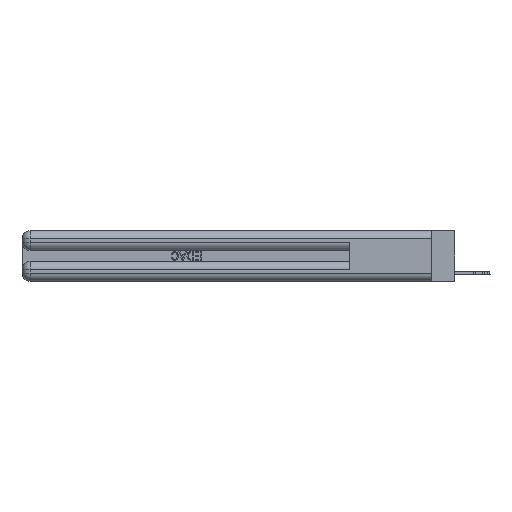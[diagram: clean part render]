
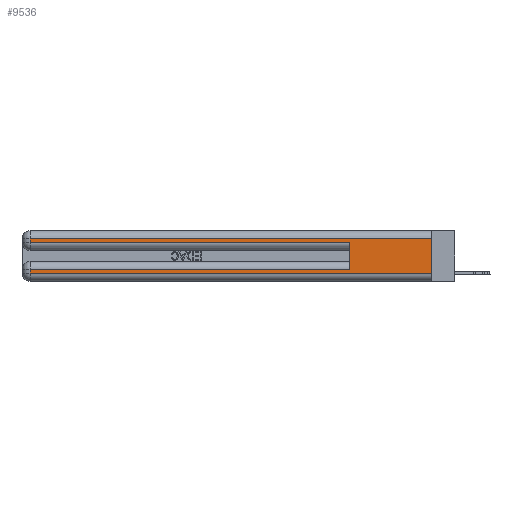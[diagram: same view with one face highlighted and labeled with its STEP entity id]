
A CAD part, left-side view. The second image highlights one B-rep face of the part: STEP entity #9536.
In plain terms, the highlighted planar face has unit normal (-1, 0, 0).
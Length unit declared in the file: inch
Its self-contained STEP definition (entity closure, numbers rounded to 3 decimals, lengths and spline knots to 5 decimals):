
#325 = DIRECTION ( 'NONE',  ( 0., -1., 0. ) ) ;
#1026 = VERTEX_POINT ( 'NONE', #5305 ) ;
#1124 = VERTEX_POINT ( 'NONE', #21292 ) ;
#1587 = CARTESIAN_POINT ( 'NONE',  ( 0., 2.94, 0.37 ) ) ;
#1974 = AXIS2_PLACEMENT_3D ( 'NONE', #2310, #13023, #29664 ) ;
#2194 = EDGE_CURVE ( 'NONE', #16568, #1026, #15857, .T. ) ;
#2310 = CARTESIAN_POINT ( 'NONE',  ( 0., 0., 0.37 ) ) ;
#2945 = LINE ( 'NONE', #22419, #12082 ) ;
#3124 = VERTEX_POINT ( 'NONE', #22089 ) ;
#4169 = ORIENTED_EDGE ( 'NONE', *, *, #14176, .T. ) ;
#4468 = VECTOR ( 'NONE', #27201, 39.37008 ) ;
#5286 = CARTESIAN_POINT ( 'NONE',  ( 0., 2.94, 0.085 ) ) ;
#5305 = CARTESIAN_POINT ( 'NONE',  ( 0., 0.6, 0.285 ) ) ;
#5596 = EDGE_CURVE ( 'NONE', #6558, #3124, #19671, .T. ) ;
#5661 = EDGE_CURVE ( 'NONE', #9516, #1124, #25423, .T. ) ;
#6558 = VERTEX_POINT ( 'NONE', #21133 ) ;
#6864 = ORIENTED_EDGE ( 'NONE', *, *, #15532, .T. ) ;
#7749 = PLANE ( 'NONE',  #1974 ) ;
#7805 = ORIENTED_EDGE ( 'NONE', *, *, #5661, .T. ) ;
#8416 = CARTESIAN_POINT ( 'NONE',  ( 0., 0., 0.06 ) ) ;
#9507 = LINE ( 'NONE', #20895, #17770 ) ;
#9516 = VERTEX_POINT ( 'NONE', #5286 ) ;
#9536 = ADVANCED_FACE ( 'NONE', ( #10735 ), #7749, .F. ) ;
#9676 = DIRECTION ( 'NONE',  ( 0., 0., 1. ) ) ;
#10185 = LINE ( 'NONE', #18909, #12363 ) ;
#10390 = ORIENTED_EDGE ( 'NONE', *, *, #20422, .T. ) ;
#10735 = FACE_OUTER_BOUND ( 'NONE', #16226, .T. ) ;
#12082 = VECTOR ( 'NONE', #325, 39.37008 ) ;
#12363 = VECTOR ( 'NONE', #29580, 39.37008 ) ;
#12465 = DIRECTION ( 'NONE',  ( 0., 0., -1. ) ) ;
#12599 = DIRECTION ( 'NONE',  ( 0., 0., -1. ) ) ;
#13023 = DIRECTION ( 'NONE',  ( 1., 0., 0. ) ) ;
#14176 = EDGE_CURVE ( 'NONE', #3124, #16568, #19188, .T. ) ;
#14536 = CARTESIAN_POINT ( 'NONE',  ( 0., 0., 0.37 ) ) ;
#15174 = CARTESIAN_POINT ( 'NONE',  ( 0., 0.6, 0.085 ) ) ;
#15532 = EDGE_CURVE ( 'NONE', #33213, #9516, #10185, .T. ) ;
#15857 = LINE ( 'NONE', #26874, #31493 ) ;
#16226 = EDGE_LOOP ( 'NONE', ( #26015, #30221, #4169, #16554, #19201, #6864, #7805, #10390 ) ) ;
#16554 = ORIENTED_EDGE ( 'NONE', *, *, #2194, .T. ) ;
#16568 = VERTEX_POINT ( 'NONE', #32295 ) ;
#17770 = VECTOR ( 'NONE', #9676, 39.37008 ) ;
#18909 = CARTESIAN_POINT ( 'NONE',  ( 0., 0., 0.085 ) ) ;
#19188 = LINE ( 'NONE', #29861, #4468 ) ;
#19201 = ORIENTED_EDGE ( 'NONE', *, *, #24202, .F. ) ;
#19671 = LINE ( 'NONE', #27002, #24826 ) ;
#20422 = EDGE_CURVE ( 'NONE', #1124, #23138, #2945, .T. ) ;
#20895 = CARTESIAN_POINT ( 'NONE',  ( 0., 0.6, 0.145 ) ) ;
#21133 = CARTESIAN_POINT ( 'NONE',  ( 0., 0., 0.31 ) ) ;
#21292 = CARTESIAN_POINT ( 'NONE',  ( 0., 2.94, 0.06 ) ) ;
#22089 = CARTESIAN_POINT ( 'NONE',  ( 0., 2.94, 0.31 ) ) ;
#22419 = CARTESIAN_POINT ( 'NONE',  ( 0., 0., 0.06 ) ) ;
#23138 = VERTEX_POINT ( 'NONE', #8416 ) ;
#23224 = EDGE_CURVE ( 'NONE', #6558, #23138, #25751, .T. ) ;
#24202 = EDGE_CURVE ( 'NONE', #33213, #1026, #9507, .T. ) ;
#24257 = DIRECTION ( 'NONE',  ( 0., -1., 0. ) ) ;
#24826 = VECTOR ( 'NONE', #30346, 39.37008 ) ;
#25423 = LINE ( 'NONE', #1587, #34371 ) ;
#25751 = LINE ( 'NONE', #14536, #29463 ) ;
#26015 = ORIENTED_EDGE ( 'NONE', *, *, #23224, .F. ) ;
#26874 = CARTESIAN_POINT ( 'NONE',  ( 0., 0., 0.285 ) ) ;
#27002 = CARTESIAN_POINT ( 'NONE',  ( 0., 0., 0.31 ) ) ;
#27201 = DIRECTION ( 'NONE',  ( 0., 0., -1. ) ) ;
#29463 = VECTOR ( 'NONE', #12599, 39.37008 ) ;
#29580 = DIRECTION ( 'NONE',  ( 0., 1., 0. ) ) ;
#29664 = DIRECTION ( 'NONE',  ( 0., 0., -1. ) ) ;
#29861 = CARTESIAN_POINT ( 'NONE',  ( 0., 2.94, 0.37 ) ) ;
#30221 = ORIENTED_EDGE ( 'NONE', *, *, #5596, .T. ) ;
#30346 = DIRECTION ( 'NONE',  ( 0., 1., 0. ) ) ;
#31493 = VECTOR ( 'NONE', #24257, 39.37008 ) ;
#32295 = CARTESIAN_POINT ( 'NONE',  ( 0., 2.94, 0.285 ) ) ;
#33213 = VERTEX_POINT ( 'NONE', #15174 ) ;
#34371 = VECTOR ( 'NONE', #12465, 39.37008 ) ;
